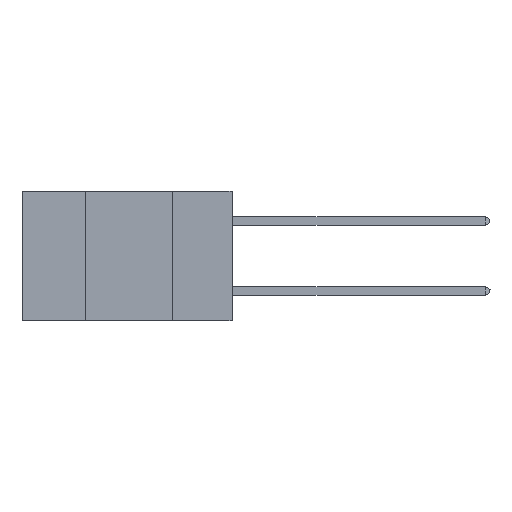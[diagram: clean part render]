
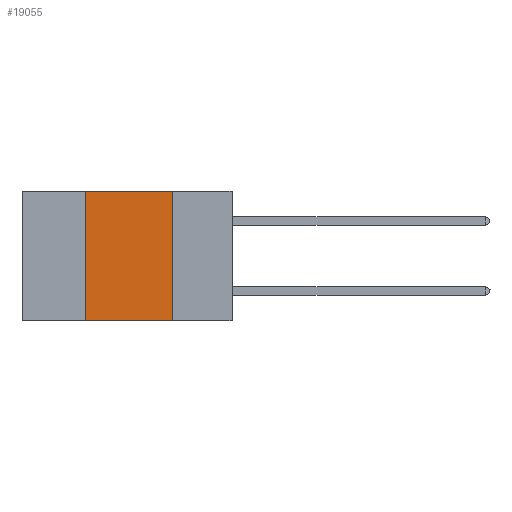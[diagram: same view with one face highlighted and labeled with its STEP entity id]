
A CAD part, left-side view. The second image highlights one B-rep face of the part: STEP entity #19055.
In plain terms, the highlighted planar face has unit normal (-1, 0, 0).
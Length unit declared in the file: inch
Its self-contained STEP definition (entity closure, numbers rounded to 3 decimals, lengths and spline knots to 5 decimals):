
#1072 = EDGE_CURVE ( 'NONE', #24336, #18655, #14469, .T. ) ;
#1501 = FACE_OUTER_BOUND ( 'NONE', #4005, .T. ) ;
#3092 = VERTEX_POINT ( 'NONE', #9615 ) ;
#3855 = CARTESIAN_POINT ( 'NONE',  ( 0., 0.17, 0. ) ) ;
#4005 = EDGE_LOOP ( 'NONE', ( #23602, #6561, #26740, #14423 ) ) ;
#4770 = DIRECTION ( 'NONE',  ( 0., -1., 0. ) ) ;
#5614 = DIRECTION ( 'NONE',  ( 0., -1., 0. ) ) ;
#5729 = DIRECTION ( 'NONE',  ( 0., 0., 1. ) ) ;
#5733 = EDGE_CURVE ( 'NONE', #24236, #18655, #17787, .T. ) ;
#6561 = ORIENTED_EDGE ( 'NONE', *, *, #20380, .F. ) ;
#7910 = VECTOR ( 'NONE', #4770, 39.37008 ) ;
#9615 = CARTESIAN_POINT ( 'NONE',  ( 0., 0.42, 0. ) ) ;
#10160 = CARTESIAN_POINT ( 'NONE',  ( 0., 0.42, -0.37 ) ) ;
#10874 = EDGE_CURVE ( 'NONE', #24236, #3092, #31581, .T. ) ;
#11541 = LINE ( 'NONE', #22148, #36549 ) ;
#12845 = PLANE ( 'NONE',  #35280 ) ;
#14423 = ORIENTED_EDGE ( 'NONE', *, *, #5733, .T. ) ;
#14469 = LINE ( 'NONE', #35766, #30842 ) ;
#17787 = LINE ( 'NONE', #17964, #7910 ) ;
#17964 = CARTESIAN_POINT ( 'NONE',  ( 0., 0.6, -0.37 ) ) ;
#18655 = VERTEX_POINT ( 'NONE', #27375 ) ;
#19055 = ADVANCED_FACE ( 'NONE', ( #1501 ), #12845, .F. ) ;
#19467 = DIRECTION ( 'NONE',  ( 0., 0., -1. ) ) ;
#20380 = EDGE_CURVE ( 'NONE', #3092, #24336, #11541, .T. ) ;
#22148 = CARTESIAN_POINT ( 'NONE',  ( 0., 0.6, 0. ) ) ;
#22256 = CARTESIAN_POINT ( 'NONE',  ( 0., 0.42, 0. ) ) ;
#22958 = VECTOR ( 'NONE', #5729, 39.37008 ) ;
#23602 = ORIENTED_EDGE ( 'NONE', *, *, #1072, .F. ) ;
#24236 = VERTEX_POINT ( 'NONE', #10160 ) ;
#24336 = VERTEX_POINT ( 'NONE', #3855 ) ;
#26740 = ORIENTED_EDGE ( 'NONE', *, *, #10874, .F. ) ;
#27375 = CARTESIAN_POINT ( 'NONE',  ( 0., 0.17, -0.37 ) ) ;
#30842 = VECTOR ( 'NONE', #39031, 39.37008 ) ;
#31581 = LINE ( 'NONE', #22256, #22958 ) ;
#35280 = AXIS2_PLACEMENT_3D ( 'NONE', #35680, #38943, #19467 ) ;
#35680 = CARTESIAN_POINT ( 'NONE',  ( 0., 0.6, 0. ) ) ;
#35766 = CARTESIAN_POINT ( 'NONE',  ( 0., 0.17, 0. ) ) ;
#36549 = VECTOR ( 'NONE', #5614, 39.37008 ) ;
#38943 = DIRECTION ( 'NONE',  ( 1., 0., 0. ) ) ;
#39031 = DIRECTION ( 'NONE',  ( 0., 0., -1. ) ) ;
